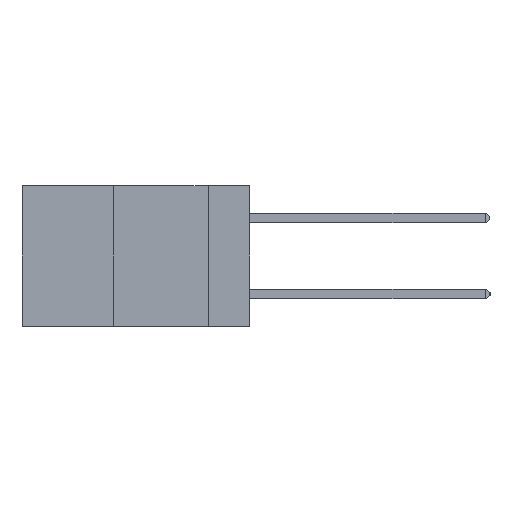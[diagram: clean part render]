
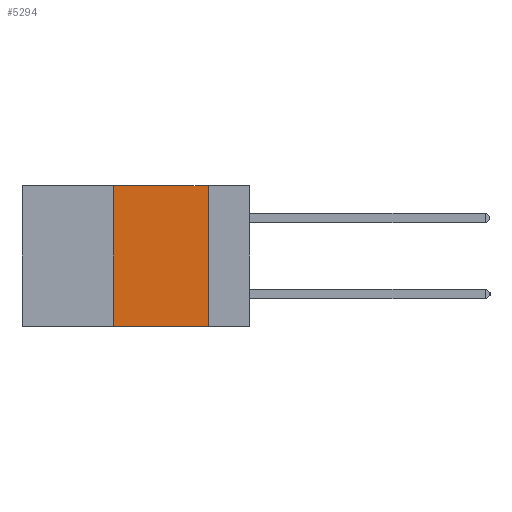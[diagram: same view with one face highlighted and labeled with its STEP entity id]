
A CAD part, left-side view. The second image highlights one B-rep face of the part: STEP entity #5294.
In plain terms, the highlighted planar face has unit normal (-1, 0, 0).
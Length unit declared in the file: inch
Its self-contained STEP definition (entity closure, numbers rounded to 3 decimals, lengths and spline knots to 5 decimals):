
#85 = CARTESIAN_POINT ( 'NONE',  ( 0., 0.6, 0. ) ) ;
#403 = CARTESIAN_POINT ( 'NONE',  ( 0., 0.6, -0.37 ) ) ;
#420 = VERTEX_POINT ( 'NONE', #5306 ) ;
#520 = LINE ( 'NONE', #403, #8196 ) ;
#646 = VERTEX_POINT ( 'NONE', #8542 ) ;
#1486 = EDGE_CURVE ( 'NONE', #8897, #4010, #7203, .T. ) ;
#1560 = DIRECTION ( 'NONE',  ( 0., 0., -1. ) ) ;
#1611 = PLANE ( 'NONE',  #7702 ) ;
#1622 = VECTOR ( 'NONE', #4449, 39.37008 ) ;
#1864 = LINE ( 'NONE', #2669, #7529 ) ;
#1951 = ORIENTED_EDGE ( 'NONE', *, *, #9232, .T. ) ;
#2289 = CARTESIAN_POINT ( 'NONE',  ( 0., 0.11, 0. ) ) ;
#2612 = CARTESIAN_POINT ( 'NONE',  ( 0., 0.11, 0. ) ) ;
#2669 = CARTESIAN_POINT ( 'NONE',  ( 0., 0.36, 0. ) ) ;
#3517 = DIRECTION ( 'NONE',  ( 0., -1., 0. ) ) ;
#3570 = EDGE_CURVE ( 'NONE', #646, #8897, #1864, .T. ) ;
#4010 = VERTEX_POINT ( 'NONE', #2612 ) ;
#4315 = DIRECTION ( 'NONE',  ( 0., -1., 0. ) ) ;
#4449 = DIRECTION ( 'NONE',  ( 0., 0., -1. ) ) ;
#5294 = ADVANCED_FACE ( 'NONE', ( #6710 ), #1611, .F. ) ;
#5306 = CARTESIAN_POINT ( 'NONE',  ( 0., 0.11, -0.37 ) ) ;
#5589 = DIRECTION ( 'NONE',  ( 0., 0., 1. ) ) ;
#5713 = ORIENTED_EDGE ( 'NONE', *, *, #1486, .F. ) ;
#5972 = LINE ( 'NONE', #2289, #1622 ) ;
#6125 = EDGE_LOOP ( 'NONE', ( #8722, #5713, #6416, #1951 ) ) ;
#6416 = ORIENTED_EDGE ( 'NONE', *, *, #3570, .F. ) ;
#6710 = FACE_OUTER_BOUND ( 'NONE', #6125, .T. ) ;
#6748 = DIRECTION ( 'NONE',  ( 1., 0., 0. ) ) ;
#7203 = LINE ( 'NONE', #8597, #7435 ) ;
#7435 = VECTOR ( 'NONE', #3517, 39.37008 ) ;
#7529 = VECTOR ( 'NONE', #5589, 39.37008 ) ;
#7702 = AXIS2_PLACEMENT_3D ( 'NONE', #85, #6748, #1560 ) ;
#8196 = VECTOR ( 'NONE', #4315, 39.37008 ) ;
#8284 = EDGE_CURVE ( 'NONE', #4010, #420, #5972, .T. ) ;
#8542 = CARTESIAN_POINT ( 'NONE',  ( 0., 0.36, -0.37 ) ) ;
#8597 = CARTESIAN_POINT ( 'NONE',  ( 0., 0.6, 0. ) ) ;
#8722 = ORIENTED_EDGE ( 'NONE', *, *, #8284, .F. ) ;
#8897 = VERTEX_POINT ( 'NONE', #9318 ) ;
#9232 = EDGE_CURVE ( 'NONE', #646, #420, #520, .T. ) ;
#9318 = CARTESIAN_POINT ( 'NONE',  ( 0., 0.36, 0. ) ) ;
